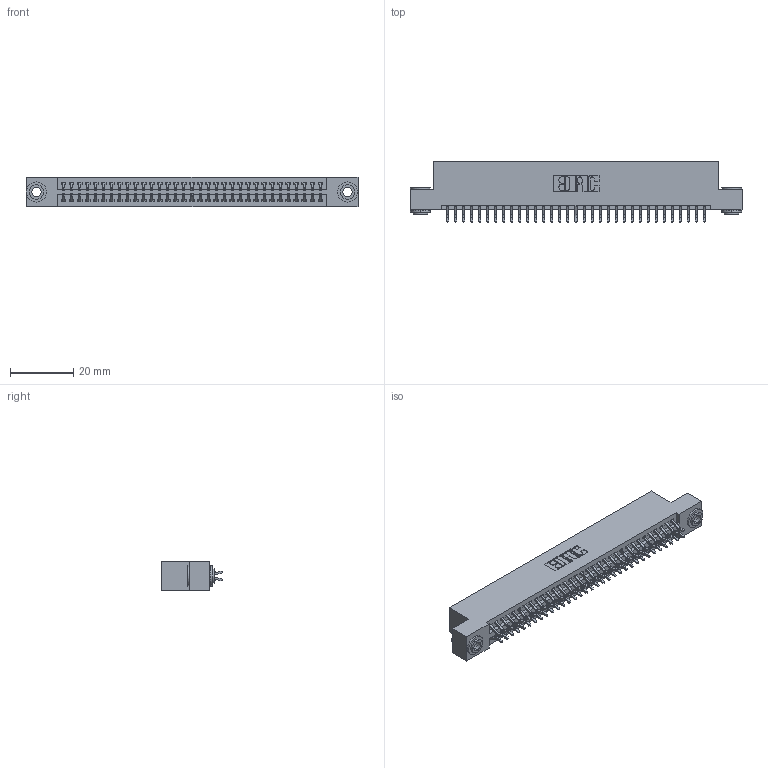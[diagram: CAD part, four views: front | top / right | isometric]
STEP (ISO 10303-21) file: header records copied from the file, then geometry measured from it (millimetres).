
FILE_DESCRIPTION (( 'STEP AP203' ), '1' );
FILE_NAME ('395-066-556-203.STEP', '2019-10-23T21:15:30', ( '' ), ( '' ), 'SwSTEP 2.0', 'SolidWorks 2016', '' );
FILE_SCHEMA (( 'CONFIG_CONTROL_DESIGN' ));
Length unit declared in the file: inch
Products named in the file (4): 345 Part_Flush Mounting Lugs - 0.156 Dia-TH; 345-292-001_556 Tail; 345-250-002_345-250-002-102; 395-066-556-203
Assembly tree (69 placements, depth 2):
  395-066-556-203
    345 Part_Flush Mounting Lugs - 0.156 Dia-TH
    345-292-001_556 Tail  x66
    345-250-002_345-250-002-102  x2
Bounding box: 105.03 x 19.24 x 9.4 mm (x, y, z)
Volume: 10135.9 mm3; surface area: 14955.3 mm2
Topology: 69 solids, 69 shells, 3860 faces, 11439 edges, 7534 vertices
Faces by surface type: plane 2532, cylinder 1320, cone 8
Entity records: 27974 total; most frequent: CARTESIAN_POINT 4687, ORIENTED_EDGE 4602, DIRECTION 4163, EDGE_CURVE 2301, LINE 2005, VECTOR 2005, VERTEX_POINT 1530, AXIS2_PLACEMENT_3D 1079
